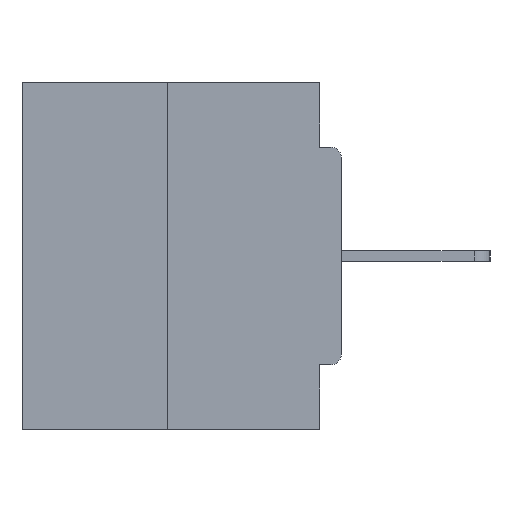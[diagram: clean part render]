
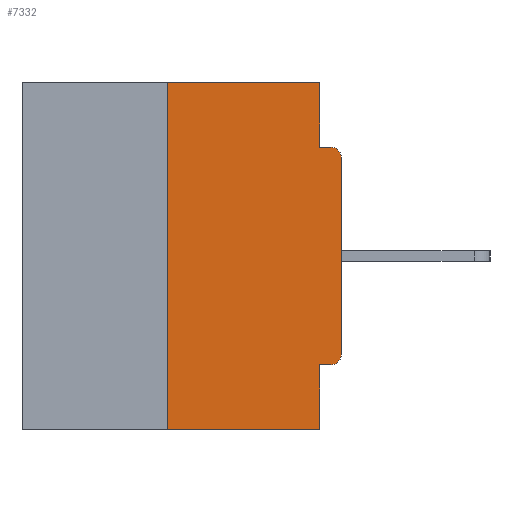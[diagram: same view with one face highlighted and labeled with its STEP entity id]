
A CAD part, left-side view. The second image highlights one B-rep face of the part: STEP entity #7332.
In plain terms, the highlighted planar face has unit normal (-1, 0, 0).
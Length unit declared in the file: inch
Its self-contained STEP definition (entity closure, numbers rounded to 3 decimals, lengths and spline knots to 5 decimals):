
#51 = LINE ( 'NONE', #19311, #14303 ) ;
#244 = LINE ( 'NONE', #9727, #21285 ) ;
#571 = LINE ( 'NONE', #10040, #26052 ) ;
#780 = CIRCLE ( 'NONE', #4208, 0.015 ) ;
#800 = DIRECTION ( 'NONE',  ( 1., 0., 0. ) ) ;
#1459 = CARTESIAN_POINT ( 'NONE',  ( 0., 0.031, -0.5 ) ) ;
#2403 = DIRECTION ( 'NONE',  ( 0., 0., 1. ) ) ;
#3224 = EDGE_CURVE ( 'NONE', #14889, #13238, #571, .T. ) ;
#3387 = CARTESIAN_POINT ( 'NONE',  ( 0., 0.031, 0. ) ) ;
#3565 = ORIENTED_EDGE ( 'NONE', *, *, #7529, .T. ) ;
#4208 = AXIS2_PLACEMENT_3D ( 'NONE', #10748, #20541, #5948 ) ;
#4878 = CARTESIAN_POINT ( 'NONE',  ( 0., 0., -0.3915 ) ) ;
#5475 = EDGE_CURVE ( 'NONE', #23792, #14889, #51, .T. ) ;
#5731 = LINE ( 'NONE', #3387, #28101 ) ;
#5746 = DIRECTION ( 'NONE',  ( 0., 0., 1. ) ) ;
#5873 = VECTOR ( 'NONE', #7714, 39.37008 ) ;
#5948 = DIRECTION ( 'NONE',  ( 0., 0., -1. ) ) ;
#6418 = CARTESIAN_POINT ( 'NONE',  ( 0., 0.015, -0.0935 ) ) ;
#6567 = ORIENTED_EDGE ( 'NONE', *, *, #15510, .T. ) ;
#6613 = CARTESIAN_POINT ( 'NONE',  ( 0., 0.031, -0.0935 ) ) ;
#6699 = VERTEX_POINT ( 'NONE', #6613 ) ;
#6720 = ORIENTED_EDGE ( 'NONE', *, *, #18824, .F. ) ;
#6724 = VERTEX_POINT ( 'NONE', #14508 ) ;
#6739 = DIRECTION ( 'NONE',  ( 0., 0., -1. ) ) ;
#6947 = VECTOR ( 'NONE', #5746, 39.37008 ) ;
#7332 = ADVANCED_FACE ( 'NONE', ( #29677 ), #17260, .F. ) ;
#7529 = EDGE_CURVE ( 'NONE', #23792, #24421, #16209, .T. ) ;
#7714 = DIRECTION ( 'NONE',  ( 0., 1., 0. ) ) ;
#8096 = EDGE_CURVE ( 'NONE', #10757, #6724, #15071, .T. ) ;
#8221 = ORIENTED_EDGE ( 'NONE', *, *, #12428, .F. ) ;
#9727 = CARTESIAN_POINT ( 'NONE',  ( 0., 0., -0.0935 ) ) ;
#9745 = CARTESIAN_POINT ( 'NONE',  ( 0., 0., -0.4065 ) ) ;
#10040 = CARTESIAN_POINT ( 'NONE',  ( 0., 0.46, 0. ) ) ;
#10748 = CARTESIAN_POINT ( 'NONE',  ( 0., 0.015, -0.3915 ) ) ;
#10757 = VERTEX_POINT ( 'NONE', #4878 ) ;
#10927 = LINE ( 'NONE', #1459, #16986 ) ;
#11006 = VERTEX_POINT ( 'NONE', #6418 ) ;
#11136 = CARTESIAN_POINT ( 'NONE',  ( 0., 0.25, 0. ) ) ;
#12037 = AXIS2_PLACEMENT_3D ( 'NONE', #17150, #29569, #12638 ) ;
#12268 = EDGE_CURVE ( 'NONE', #6724, #11006, #25928, .T. ) ;
#12428 = EDGE_CURVE ( 'NONE', #20900, #24421, #10927, .T. ) ;
#12638 = DIRECTION ( 'NONE',  ( 0., 0., -1. ) ) ;
#12894 = DIRECTION ( 'NONE',  ( 0., 0., -1. ) ) ;
#12914 = ORIENTED_EDGE ( 'NONE', *, *, #3224, .F. ) ;
#13025 = CARTESIAN_POINT ( 'NONE',  ( 0., 0.031, 0. ) ) ;
#13238 = VERTEX_POINT ( 'NONE', #13025 ) ;
#14303 = VECTOR ( 'NONE', #2403, 39.37008 ) ;
#14508 = CARTESIAN_POINT ( 'NONE',  ( 0., 0., -0.1085 ) ) ;
#14889 = VERTEX_POINT ( 'NONE', #11136 ) ;
#15071 = LINE ( 'NONE', #24689, #6947 ) ;
#15170 = VERTEX_POINT ( 'NONE', #26492 ) ;
#15510 = EDGE_CURVE ( 'NONE', #15170, #10757, #780, .T. ) ;
#16209 = LINE ( 'NONE', #20571, #19808 ) ;
#16986 = VECTOR ( 'NONE', #6739, 39.37008 ) ;
#17046 = LINE ( 'NONE', #9745, #5873 ) ;
#17150 = CARTESIAN_POINT ( 'NONE',  ( 0., 0.015, -0.1085 ) ) ;
#17260 = PLANE ( 'NONE',  #18839 ) ;
#18571 = CARTESIAN_POINT ( 'NONE',  ( 0., 0.031, -0.4065 ) ) ;
#18824 = EDGE_CURVE ( 'NONE', #13238, #6699, #5731, .T. ) ;
#18839 = AXIS2_PLACEMENT_3D ( 'NONE', #27199, #800, #12894 ) ;
#19311 = CARTESIAN_POINT ( 'NONE',  ( 0., 0.25, 0. ) ) ;
#19516 = DIRECTION ( 'NONE',  ( 0., -1., 0. ) ) ;
#19540 = CARTESIAN_POINT ( 'NONE',  ( 0., 0.031, -0.5 ) ) ;
#19644 = ORIENTED_EDGE ( 'NONE', *, *, #5475, .F. ) ;
#19808 = VECTOR ( 'NONE', #25688, 39.37008 ) ;
#19949 = CARTESIAN_POINT ( 'NONE',  ( 0., 0.25, -0.5 ) ) ;
#20174 = ORIENTED_EDGE ( 'NONE', *, *, #20751, .F. ) ;
#20541 = DIRECTION ( 'NONE',  ( -1., 0., 0. ) ) ;
#20546 = ORIENTED_EDGE ( 'NONE', *, *, #12268, .T. ) ;
#20571 = CARTESIAN_POINT ( 'NONE',  ( 0., 0.46, -0.5 ) ) ;
#20751 = EDGE_CURVE ( 'NONE', #15170, #20900, #17046, .T. ) ;
#20900 = VERTEX_POINT ( 'NONE', #18571 ) ;
#21285 = VECTOR ( 'NONE', #28982, 39.37008 ) ;
#23649 = EDGE_CURVE ( 'NONE', #6699, #11006, #244, .T. ) ;
#23792 = VERTEX_POINT ( 'NONE', #19949 ) ;
#24173 = EDGE_LOOP ( 'NONE', ( #12914, #19644, #3565, #8221, #20174, #6567, #29210, #20546, #25419, #6720 ) ) ;
#24421 = VERTEX_POINT ( 'NONE', #19540 ) ;
#24689 = CARTESIAN_POINT ( 'NONE',  ( 0., 0., 0. ) ) ;
#25419 = ORIENTED_EDGE ( 'NONE', *, *, #23649, .F. ) ;
#25688 = DIRECTION ( 'NONE',  ( 0., -1., 0. ) ) ;
#25928 = CIRCLE ( 'NONE', #12037, 0.015 ) ;
#26052 = VECTOR ( 'NONE', #19516, 39.37008 ) ;
#26492 = CARTESIAN_POINT ( 'NONE',  ( 0., 0.015, -0.4065 ) ) ;
#27199 = CARTESIAN_POINT ( 'NONE',  ( 0., 0.46, 0. ) ) ;
#28101 = VECTOR ( 'NONE', #29027, 39.37008 ) ;
#28982 = DIRECTION ( 'NONE',  ( 0., -1., 0. ) ) ;
#29027 = DIRECTION ( 'NONE',  ( 0., 0., -1. ) ) ;
#29210 = ORIENTED_EDGE ( 'NONE', *, *, #8096, .T. ) ;
#29569 = DIRECTION ( 'NONE',  ( -1., 0., 0. ) ) ;
#29677 = FACE_OUTER_BOUND ( 'NONE', #24173, .T. ) ;
